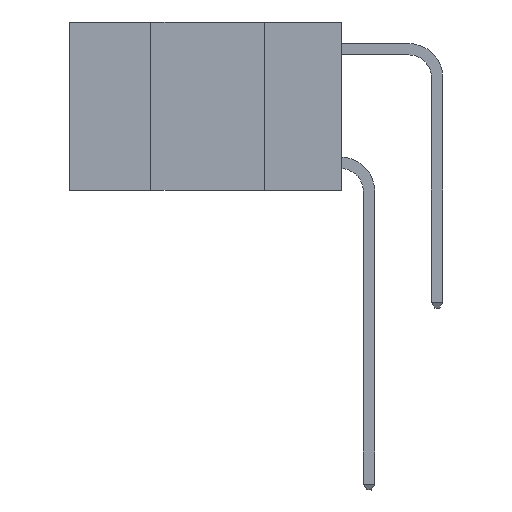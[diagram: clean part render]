
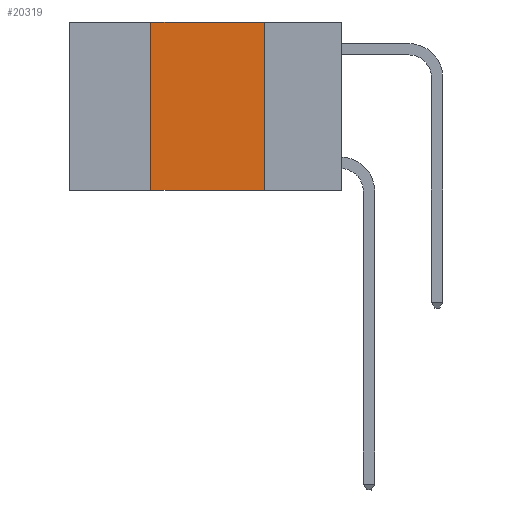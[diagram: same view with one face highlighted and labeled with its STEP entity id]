
A CAD part, left-side view. The second image highlights one B-rep face of the part: STEP entity #20319.
In plain terms, the highlighted planar face has unit normal (-1, 0, 0).
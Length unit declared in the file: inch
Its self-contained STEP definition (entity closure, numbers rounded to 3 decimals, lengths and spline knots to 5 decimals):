
#888 = VECTOR ( 'NONE', #12100, 39.37008 ) ;
#1005 = ORIENTED_EDGE ( 'NONE', *, *, #12336, .T. ) ;
#1052 = CARTESIAN_POINT ( 'NONE',  ( 0., 0.42, -0.37 ) ) ;
#1255 = CARTESIAN_POINT ( 'NONE',  ( 0., 0.42, 0. ) ) ;
#1414 = FACE_OUTER_BOUND ( 'NONE', #24058, .T. ) ;
#1656 = EDGE_CURVE ( 'NONE', #22472, #6603, #9155, .T. ) ;
#2876 = VERTEX_POINT ( 'NONE', #7466 ) ;
#2995 = EDGE_CURVE ( 'NONE', #6603, #22009, #10285, .T. ) ;
#5190 = ORIENTED_EDGE ( 'NONE', *, *, #1656, .F. ) ;
#6603 = VERTEX_POINT ( 'NONE', #7547 ) ;
#6817 = DIRECTION ( 'NONE',  ( 0., 0., 1. ) ) ;
#6843 = DIRECTION ( 'NONE',  ( 1., 0., 0. ) ) ;
#7466 = CARTESIAN_POINT ( 'NONE',  ( 0., 0.17, -0.37 ) ) ;
#7547 = CARTESIAN_POINT ( 'NONE',  ( 0., 0.42, 0. ) ) ;
#7672 = DIRECTION ( 'NONE',  ( 0., 0., -1. ) ) ;
#8982 = PLANE ( 'NONE',  #11430 ) ;
#9155 = LINE ( 'NONE', #1255, #21794 ) ;
#10114 = EDGE_CURVE ( 'NONE', #22009, #2876, #16646, .T. ) ;
#10285 = LINE ( 'NONE', #21337, #888 ) ;
#11430 = AXIS2_PLACEMENT_3D ( 'NONE', #16308, #6843, #12713 ) ;
#11665 = VECTOR ( 'NONE', #7672, 39.37008 ) ;
#12100 = DIRECTION ( 'NONE',  ( 0., -1., 0. ) ) ;
#12112 = LINE ( 'NONE', #19524, #23850 ) ;
#12336 = EDGE_CURVE ( 'NONE', #22472, #2876, #12112, .T. ) ;
#12713 = DIRECTION ( 'NONE',  ( 0., 0., -1. ) ) ;
#15662 = ORIENTED_EDGE ( 'NONE', *, *, #2995, .F. ) ;
#16308 = CARTESIAN_POINT ( 'NONE',  ( 0., 0.6, 0. ) ) ;
#16646 = LINE ( 'NONE', #18744, #11665 ) ;
#16833 = CARTESIAN_POINT ( 'NONE',  ( 0., 0.17, 0. ) ) ;
#18744 = CARTESIAN_POINT ( 'NONE',  ( 0., 0.17, 0. ) ) ;
#19524 = CARTESIAN_POINT ( 'NONE',  ( 0., 0.6, -0.37 ) ) ;
#20319 = ADVANCED_FACE ( 'NONE', ( #1414 ), #8982, .F. ) ;
#21337 = CARTESIAN_POINT ( 'NONE',  ( 0., 0.6, 0. ) ) ;
#21794 = VECTOR ( 'NONE', #6817, 39.37008 ) ;
#21969 = DIRECTION ( 'NONE',  ( 0., -1., 0. ) ) ;
#22009 = VERTEX_POINT ( 'NONE', #16833 ) ;
#22472 = VERTEX_POINT ( 'NONE', #1052 ) ;
#22952 = ORIENTED_EDGE ( 'NONE', *, *, #10114, .F. ) ;
#23850 = VECTOR ( 'NONE', #21969, 39.37008 ) ;
#24058 = EDGE_LOOP ( 'NONE', ( #22952, #15662, #5190, #1005 ) ) ;
